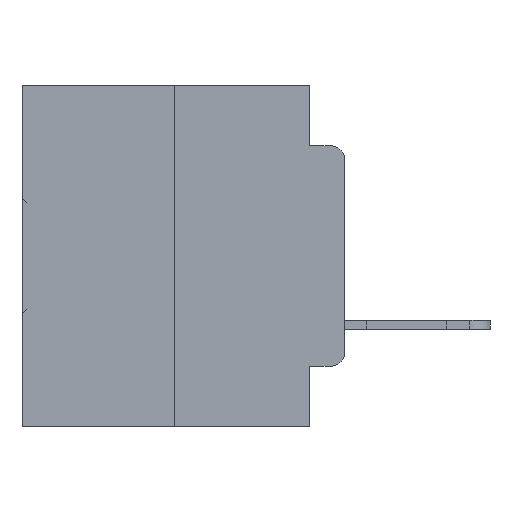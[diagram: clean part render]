
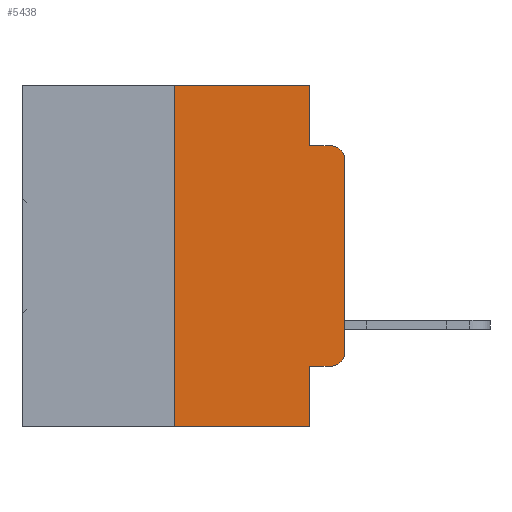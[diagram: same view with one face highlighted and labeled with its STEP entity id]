
A CAD part, left-side view. The second image highlights one B-rep face of the part: STEP entity #5438.
In plain terms, the highlighted planar face has unit normal (-1, 0, 0).
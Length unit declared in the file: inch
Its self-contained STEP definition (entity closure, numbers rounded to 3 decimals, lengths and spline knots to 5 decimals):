
#902 = AXIS2_PLACEMENT_3D ( 'NONE', #19648, #19619, #19543 ) ;
#1328 = CARTESIAN_POINT ( 'NONE',  ( 0., 0.25, 0. ) ) ;
#1542 = EDGE_CURVE ( 'NONE', #29289, #7129, #16124, .T. ) ;
#1782 = LINE ( 'NONE', #26228, #22096 ) ;
#2279 = CARTESIAN_POINT ( 'NONE',  ( 0., 0.051, -0.0885 ) ) ;
#3157 = PLANE ( 'NONE',  #28760 ) ;
#3316 = CARTESIAN_POINT ( 'NONE',  ( 0., 0.473, 0. ) ) ;
#3453 = CARTESIAN_POINT ( 'NONE',  ( 0., 0.051, -0.5 ) ) ;
#3756 = CARTESIAN_POINT ( 'NONE',  ( 0., 0.02, -0.0885 ) ) ;
#3962 = ORIENTED_EDGE ( 'NONE', *, *, #14756, .F. ) ;
#4563 = VERTEX_POINT ( 'NONE', #24876 ) ;
#5438 = ADVANCED_FACE ( 'NONE', ( #9734 ), #3157, .F. ) ;
#5479 = VECTOR ( 'NONE', #21230, 39.37008 ) ;
#6326 = LINE ( 'NONE', #22926, #19718 ) ;
#6954 = AXIS2_PLACEMENT_3D ( 'NONE', #26227, #26141, #25921 ) ;
#7109 = ORIENTED_EDGE ( 'NONE', *, *, #1542, .F. ) ;
#7129 = VERTEX_POINT ( 'NONE', #26196 ) ;
#7538 = VERTEX_POINT ( 'NONE', #31690 ) ;
#7679 = CARTESIAN_POINT ( 'NONE',  ( 0., 0.02, -0.4115 ) ) ;
#8178 = VECTOR ( 'NONE', #30423, 39.37008 ) ;
#9734 = FACE_OUTER_BOUND ( 'NONE', #19154, .T. ) ;
#10597 = VECTOR ( 'NONE', #27865, 39.37008 ) ;
#11860 = LINE ( 'NONE', #21274, #5479 ) ;
#12615 = ORIENTED_EDGE ( 'NONE', *, *, #14664, .F. ) ;
#14102 = EDGE_CURVE ( 'NONE', #4563, #31571, #22554, .T. ) ;
#14620 = EDGE_CURVE ( 'NONE', #21466, #17001, #17653, .T. ) ;
#14661 = EDGE_CURVE ( 'NONE', #17001, #30065, #16011, .T. ) ;
#14664 = EDGE_CURVE ( 'NONE', #32216, #30065, #1782, .T. ) ;
#14702 = EDGE_CURVE ( 'NONE', #7129, #32216, #20543, .T. ) ;
#14712 = EDGE_CURVE ( 'NONE', #4563, #29289, #6326, .T. ) ;
#14756 = EDGE_CURVE ( 'NONE', #7538, #31571, #11860, .T. ) ;
#14768 = EDGE_CURVE ( 'NONE', #7538, #16713, #24824, .T. ) ;
#14775 = EDGE_CURVE ( 'NONE', #16713, #21466, #30305, .T. ) ;
#16011 = CIRCLE ( 'NONE', #6954, 0.02 ) ;
#16124 = LINE ( 'NONE', #22220, #8178 ) ;
#16713 = VERTEX_POINT ( 'NONE', #7679 ) ;
#17001 = VERTEX_POINT ( 'NONE', #31649 ) ;
#17653 = LINE ( 'NONE', #28322, #10597 ) ;
#18887 = VECTOR ( 'NONE', #20425, 39.37008 ) ;
#19154 = EDGE_LOOP ( 'NONE', ( #23230, #26765, #12615, #26280, #7109, #32036, #28903, #3962, #31698, #27442 ) ) ;
#19543 = DIRECTION ( 'NONE',  ( 0., 0., -1. ) ) ;
#19619 = DIRECTION ( 'NONE',  ( -1., 0., 0. ) ) ;
#19648 = CARTESIAN_POINT ( 'NONE',  ( 0., 0.02, -0.3915 ) ) ;
#19718 = VECTOR ( 'NONE', #22770, 39.37008 ) ;
#20425 = DIRECTION ( 'NONE',  ( 0., -1., 0. ) ) ;
#20543 = LINE ( 'NONE', #23364, #21341 ) ;
#20732 = CARTESIAN_POINT ( 'NONE',  ( 0., 0.051, -0.4115 ) ) ;
#21230 = DIRECTION ( 'NONE',  ( 0., 0., -1. ) ) ;
#21274 = CARTESIAN_POINT ( 'NONE',  ( 0., 0.051, 0. ) ) ;
#21341 = VECTOR ( 'NONE', #23357, 39.37008 ) ;
#21466 = VERTEX_POINT ( 'NONE', #31355 ) ;
#22096 = VECTOR ( 'NONE', #26586, 39.37008 ) ;
#22220 = CARTESIAN_POINT ( 'NONE',  ( 0., 0.473, 0. ) ) ;
#22293 = DIRECTION ( 'NONE',  ( 0., -1., 0. ) ) ;
#22375 = DIRECTION ( 'NONE',  ( 0., 0., -1. ) ) ;
#22554 = LINE ( 'NONE', #23645, #28230 ) ;
#22770 = DIRECTION ( 'NONE',  ( 0., 0., 1. ) ) ;
#22926 = CARTESIAN_POINT ( 'NONE',  ( 0., 0.25, 0. ) ) ;
#23230 = ORIENTED_EDGE ( 'NONE', *, *, #14620, .T. ) ;
#23357 = DIRECTION ( 'NONE',  ( 0., 0., -1. ) ) ;
#23364 = CARTESIAN_POINT ( 'NONE',  ( 0., 0.051, 0. ) ) ;
#23645 = CARTESIAN_POINT ( 'NONE',  ( 0., 0.473, -0.5 ) ) ;
#24824 = LINE ( 'NONE', #20732, #18887 ) ;
#24876 = CARTESIAN_POINT ( 'NONE',  ( 0., 0.25, -0.5 ) ) ;
#25921 = DIRECTION ( 'NONE',  ( 0., 0., -1. ) ) ;
#26141 = DIRECTION ( 'NONE',  ( -1., 0., 0. ) ) ;
#26196 = CARTESIAN_POINT ( 'NONE',  ( 0., 0.051, 0. ) ) ;
#26227 = CARTESIAN_POINT ( 'NONE',  ( 0., 0.02, -0.1085 ) ) ;
#26228 = CARTESIAN_POINT ( 'NONE',  ( 0., 0.051, -0.0885 ) ) ;
#26280 = ORIENTED_EDGE ( 'NONE', *, *, #14702, .F. ) ;
#26586 = DIRECTION ( 'NONE',  ( 0., -1., 0. ) ) ;
#26634 = DIRECTION ( 'NONE',  ( 1., 0., 0. ) ) ;
#26765 = ORIENTED_EDGE ( 'NONE', *, *, #14661, .T. ) ;
#27442 = ORIENTED_EDGE ( 'NONE', *, *, #14775, .T. ) ;
#27865 = DIRECTION ( 'NONE',  ( 0., 0., 1. ) ) ;
#28230 = VECTOR ( 'NONE', #22293, 39.37008 ) ;
#28322 = CARTESIAN_POINT ( 'NONE',  ( 0., 0., 0. ) ) ;
#28760 = AXIS2_PLACEMENT_3D ( 'NONE', #3316, #26634, #22375 ) ;
#28903 = ORIENTED_EDGE ( 'NONE', *, *, #14102, .T. ) ;
#29289 = VERTEX_POINT ( 'NONE', #1328 ) ;
#30065 = VERTEX_POINT ( 'NONE', #3756 ) ;
#30305 = CIRCLE ( 'NONE', #902, 0.02 ) ;
#30423 = DIRECTION ( 'NONE',  ( 0., -1., 0. ) ) ;
#31355 = CARTESIAN_POINT ( 'NONE',  ( 0., 0., -0.3915 ) ) ;
#31571 = VERTEX_POINT ( 'NONE', #3453 ) ;
#31649 = CARTESIAN_POINT ( 'NONE',  ( 0., 0., -0.1085 ) ) ;
#31690 = CARTESIAN_POINT ( 'NONE',  ( 0., 0.051, -0.4115 ) ) ;
#31698 = ORIENTED_EDGE ( 'NONE', *, *, #14768, .T. ) ;
#32036 = ORIENTED_EDGE ( 'NONE', *, *, #14712, .F. ) ;
#32216 = VERTEX_POINT ( 'NONE', #2279 ) ;
